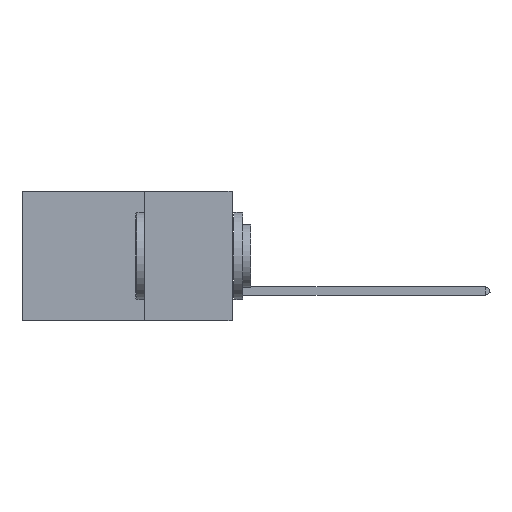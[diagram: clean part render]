
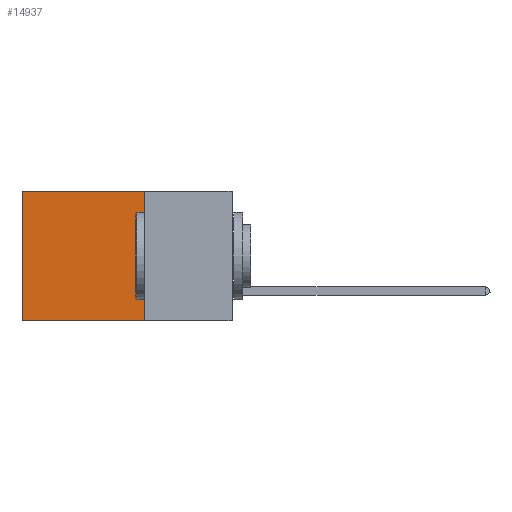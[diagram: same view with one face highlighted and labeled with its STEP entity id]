
A CAD part, left-side view. The second image highlights one B-rep face of the part: STEP entity #14937.
In plain terms, the highlighted planar face has unit normal (-1, 0, 0).
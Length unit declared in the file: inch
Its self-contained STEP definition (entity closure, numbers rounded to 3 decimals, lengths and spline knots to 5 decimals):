
#516 = VERTEX_POINT ( 'NONE', #10737 ) ;
#1510 = EDGE_CURVE ( 'NONE', #8604, #8506, #9689, .T. ) ;
#1937 = LINE ( 'NONE', #9955, #8233 ) ;
#1980 = ORIENTED_EDGE ( 'NONE', *, *, #8492, .F. ) ;
#2055 = ORIENTED_EDGE ( 'NONE', *, *, #13930, .T. ) ;
#2159 = DIRECTION ( 'NONE',  ( 0., 1., 0. ) ) ;
#2571 = FACE_OUTER_BOUND ( 'NONE', #10983, .T. ) ;
#2581 = CARTESIAN_POINT ( 'NONE',  ( 0.2875, 0.25, 0. ) ) ;
#2911 = ORIENTED_EDGE ( 'NONE', *, *, #15188, .T. ) ;
#3143 = PLANE ( 'NONE',  #10954 ) ;
#3302 = DIRECTION ( 'NONE',  ( 0., 0., -1. ) ) ;
#3587 = VERTEX_POINT ( 'NONE', #2581 ) ;
#4136 = VECTOR ( 'NONE', #13030, 39.37008 ) ;
#4780 = CARTESIAN_POINT ( 'NONE',  ( 0.2875, 0.25, 0. ) ) ;
#7213 = CARTESIAN_POINT ( 'NONE',  ( 0.2875, 0.25, -0.37 ) ) ;
#7273 = DIRECTION ( 'NONE',  ( 1., 0., 0. ) ) ;
#8233 = VECTOR ( 'NONE', #3302, 39.37008 ) ;
#8429 = VECTOR ( 'NONE', #2159, 39.37008 ) ;
#8492 = EDGE_CURVE ( 'NONE', #3587, #8604, #15479, .T. ) ;
#8506 = VERTEX_POINT ( 'NONE', #15745 ) ;
#8604 = VERTEX_POINT ( 'NONE', #7213 ) ;
#8726 = LINE ( 'NONE', #9789, #12682 ) ;
#9383 = ORIENTED_EDGE ( 'NONE', *, *, #1510, .F. ) ;
#9689 = LINE ( 'NONE', #16788, #8429 ) ;
#9789 = CARTESIAN_POINT ( 'NONE',  ( 0.2875, 0.25, 0. ) ) ;
#9955 = CARTESIAN_POINT ( 'NONE',  ( 0.2875, 0.6, 0. ) ) ;
#10737 = CARTESIAN_POINT ( 'NONE',  ( 0.2875, 0.6, 0. ) ) ;
#10954 = AXIS2_PLACEMENT_3D ( 'NONE', #12535, #7273, #14077 ) ;
#10983 = EDGE_LOOP ( 'NONE', ( #2911, #9383, #1980, #2055 ) ) ;
#11318 = DIRECTION ( 'NONE',  ( 0., 1., 0. ) ) ;
#12535 = CARTESIAN_POINT ( 'NONE',  ( 0.2875, 0.25, 0. ) ) ;
#12682 = VECTOR ( 'NONE', #11318, 39.37008 ) ;
#13030 = DIRECTION ( 'NONE',  ( 0., 0., -1. ) ) ;
#13930 = EDGE_CURVE ( 'NONE', #3587, #516, #8726, .T. ) ;
#14077 = DIRECTION ( 'NONE',  ( 0., 0., -1. ) ) ;
#14937 = ADVANCED_FACE ( 'NONE', ( #2571 ), #3143, .F. ) ;
#15188 = EDGE_CURVE ( 'NONE', #516, #8506, #1937, .T. ) ;
#15479 = LINE ( 'NONE', #4780, #4136 ) ;
#15745 = CARTESIAN_POINT ( 'NONE',  ( 0.2875, 0.6, -0.37 ) ) ;
#16788 = CARTESIAN_POINT ( 'NONE',  ( 0.2875, 0.25, -0.37 ) ) ;
